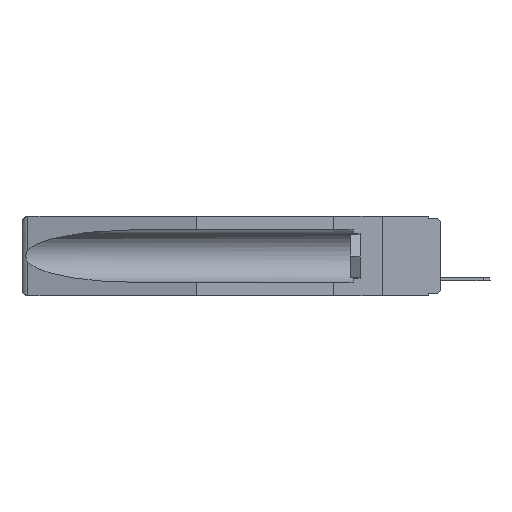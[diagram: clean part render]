
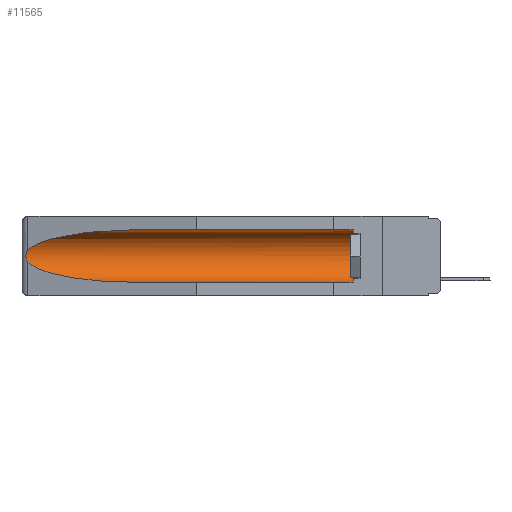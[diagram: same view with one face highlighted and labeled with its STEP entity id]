
A CAD part, left-side view. The second image highlights one B-rep face of the part: STEP entity #11565.
In plain terms, the highlighted cylindrical face has radius 2.857 mm (diameter 5.715 mm), a partial arc.
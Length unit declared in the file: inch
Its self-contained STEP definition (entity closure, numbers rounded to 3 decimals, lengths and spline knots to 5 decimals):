
#716 = CARTESIAN_POINT ( 'NONE',  ( 0.2675, 1.53308, -0.17534 ) ) ;
#1170 = VECTOR ( 'NONE', #1623, 39.37008 ) ;
#1610 =( BOUNDED_CURVE ( )  B_SPLINE_CURVE ( 3, ( #7033, #16130, #12113, #13373 ),
 .UNSPECIFIED., .F., .T. ) 
 B_SPLINE_CURVE_WITH_KNOTS ( ( 4, 4 ),
 ( 4.71239, 6.08839 ),
 .UNSPECIFIED. ) 
 CURVE ( )  GEOMETRIC_REPRESENTATION_ITEM ( )  RATIONAL_B_SPLINE_CURVE ( ( 1., 0.848, 0.848, 1. ) ) 
 REPRESENTATION_ITEM ( '' )  );
#1623 = DIRECTION ( 'NONE',  ( 0., 1., 0. ) ) ;
#2140 = CARTESIAN_POINT ( 'NONE',  ( 0.26597, 1.5296, -0.19026 ) ) ;
#2383 = VERTEX_POINT ( 'NONE', #3987 ) ;
#2525 = CARTESIAN_POINT ( 'NONE',  ( 0.155, 0.126, -0.1715 ) ) ;
#2661 = CARTESIAN_POINT ( 'NONE',  ( 0.155, 0.126, -0.059 ) ) ;
#2679 = CARTESIAN_POINT ( 'NONE',  ( 0.155, 0.126, -0.284 ) ) ;
#2842 = EDGE_CURVE ( 'NONE', #12043, #4312, #9220, .T. ) ;
#3047 = VERTEX_POINT ( 'NONE', #3135 ) ;
#3135 = CARTESIAN_POINT ( 'NONE',  ( 0.26537, 1.52718, -0.14972 ) ) ;
#3469 = ORIENTED_EDGE ( 'NONE', *, *, #11514, .T. ) ;
#3858 = DIRECTION ( 'NONE',  ( 0., -1., 0. ) ) ;
#3898 = EDGE_LOOP ( 'NONE', ( #16170, #13482, #13689, #6797, #4102, #3469 ) ) ;
#3987 = CARTESIAN_POINT ( 'NONE',  ( 0.26537, 1.52718, -0.19328 ) ) ;
#4102 = ORIENTED_EDGE ( 'NONE', *, *, #16102, .T. ) ;
#4303 = EDGE_CURVE ( 'NONE', #3047, #2383, #14264, .T. ) ;
#4312 = VERTEX_POINT ( 'NONE', #5955 ) ;
#4653 = EDGE_CURVE ( 'NONE', #13572, #3047, #1610, .T. ) ;
#5150 = CARTESIAN_POINT ( 'NONE',  ( 0.155, 1.07973, -0.059 ) ) ;
#5274 = DIRECTION ( 'NONE',  ( 0., 1., 0. ) ) ;
#5434 = FACE_OUTER_BOUND ( 'NONE', #3898, .T. ) ;
#5520 = VECTOR ( 'NONE', #6735, 39.37008 ) ;
#5636 = CARTESIAN_POINT ( 'NONE',  ( 0.2673, 1.53269, -0.17917 ) ) ;
#5955 = CARTESIAN_POINT ( 'NONE',  ( 0.155, 1.07973, -0.284 ) ) ;
#6093 = AXIS2_PLACEMENT_3D ( 'NONE', #2525, #3858, #10348 ) ;
#6735 = DIRECTION ( 'NONE',  ( 0., 1., 0. ) ) ;
#6797 = ORIENTED_EDGE ( 'NONE', *, *, #2842, .F. ) ;
#7033 = CARTESIAN_POINT ( 'NONE',  ( 0.155, 1.07973, -0.059 ) ) ;
#7217 = CARTESIAN_POINT ( 'NONE',  ( 0.26537, 1.52718, -0.19328 ) ) ;
#7767 = CYLINDRICAL_SURFACE ( 'NONE', #11446, 0.1125 ) ;
#7977 = CARTESIAN_POINT ( 'NONE',  ( 0.155, -0.30754, -0.284 ) ) ;
#9096 = EDGE_CURVE ( 'NONE', #2383, #4312, #13180, .T. ) ;
#9186 = CARTESIAN_POINT ( 'NONE',  ( 0.155, -0.30754, -0.059 ) ) ;
#9220 = LINE ( 'NONE', #7977, #5520 ) ;
#10348 = DIRECTION ( 'NONE',  ( 0., 0., 1. ) ) ;
#10467 = CARTESIAN_POINT ( 'NONE',  ( 0.25451, 1.48313, -0.24835 ) ) ;
#10509 = CARTESIAN_POINT ( 'NONE',  ( 0.155, -0.30754, -0.1715 ) ) ;
#10608 = CIRCLE ( 'NONE', #6093, 0.1125 ) ;
#11026 = CARTESIAN_POINT ( 'NONE',  ( 0.2673, 1.5327, -0.16383 ) ) ;
#11446 = AXIS2_PLACEMENT_3D ( 'NONE', #10509, #5274, #12863 ) ;
#11514 = EDGE_CURVE ( 'NONE', #13666, #13572, #15639, .T. ) ;
#11565 = ADVANCED_FACE ( 'NONE', ( #5434 ), #7767, .F. ) ;
#11807 = CARTESIAN_POINT ( 'NONE',  ( 0.21114, 1.30732, -0.284 ) ) ;
#11983 = CARTESIAN_POINT ( 'NONE',  ( 0.26654, 1.53092, -0.15636 ) ) ;
#12043 = VERTEX_POINT ( 'NONE', #2679 ) ;
#12113 = CARTESIAN_POINT ( 'NONE',  ( 0.25451, 1.48313, -0.09465 ) ) ;
#12132 = CARTESIAN_POINT ( 'NONE',  ( 0.2675, 1.53308, -0.16763 ) ) ;
#12863 = DIRECTION ( 'NONE',  ( 0., 0., 1. ) ) ;
#13180 =( BOUNDED_CURVE ( )  B_SPLINE_CURVE ( 3, ( #13980, #10467, #11807, #15513 ),
 .UNSPECIFIED., .F., .F. ) 
 B_SPLINE_CURVE_WITH_KNOTS ( ( 4, 4 ),
 ( 0.1948, 1.5708 ),
 .UNSPECIFIED. ) 
 CURVE ( )  GEOMETRIC_REPRESENTATION_ITEM ( )  RATIONAL_B_SPLINE_CURVE ( ( 1., 0.848, 0.848, 1. ) ) 
 REPRESENTATION_ITEM ( '' )  );
#13316 = CARTESIAN_POINT ( 'NONE',  ( 0.26655, 1.53094, -0.18657 ) ) ;
#13373 = CARTESIAN_POINT ( 'NONE',  ( 0.26537, 1.52718, -0.14972 ) ) ;
#13482 = ORIENTED_EDGE ( 'NONE', *, *, #4303, .T. ) ;
#13562 = CARTESIAN_POINT ( 'NONE',  ( 0.26537, 1.52718, -0.14972 ) ) ;
#13572 = VERTEX_POINT ( 'NONE', #5150 ) ;
#13666 = VERTEX_POINT ( 'NONE', #2661 ) ;
#13689 = ORIENTED_EDGE ( 'NONE', *, *, #9096, .T. ) ;
#13980 = CARTESIAN_POINT ( 'NONE',  ( 0.26537, 1.52718, -0.19328 ) ) ;
#14264 = B_SPLINE_CURVE_WITH_KNOTS ( 'NONE', 3,
 ( #13562, #16073, #11983, #11026, #12132, #716, #5636, #13316, #2140, #7217 ),
 .UNSPECIFIED., .F., .F.,
 ( 4, 2, 2, 2, 4 ),
 ( 0., 0.00029, 0.00058, 0.00087, 0.00117 ),
 .UNSPECIFIED. ) ;
#15513 = CARTESIAN_POINT ( 'NONE',  ( 0.155, 1.07973, -0.284 ) ) ;
#15639 = LINE ( 'NONE', #9186, #1170 ) ;
#16073 = CARTESIAN_POINT ( 'NONE',  ( 0.26597, 1.52961, -0.15275 ) ) ;
#16102 = EDGE_CURVE ( 'NONE', #12043, #13666, #10608, .T. ) ;
#16130 = CARTESIAN_POINT ( 'NONE',  ( 0.21114, 1.30732, -0.059 ) ) ;
#16170 = ORIENTED_EDGE ( 'NONE', *, *, #4653, .T. ) ;
